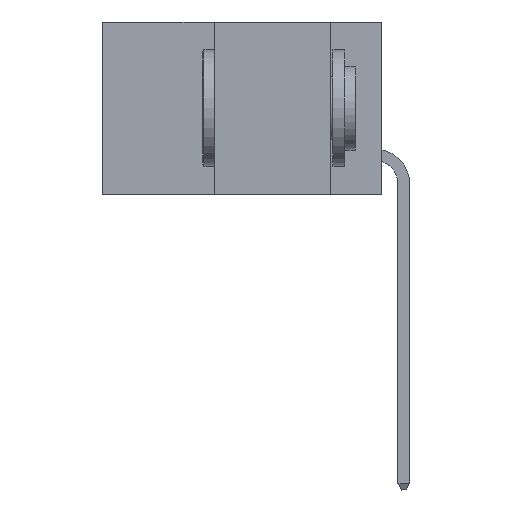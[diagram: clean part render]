
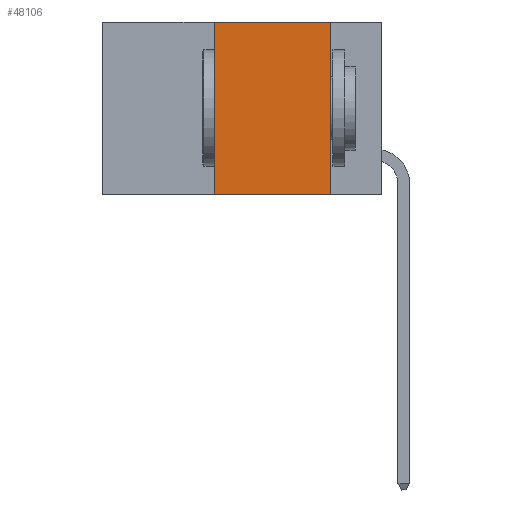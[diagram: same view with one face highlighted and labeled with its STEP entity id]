
A CAD part, left-side view. The second image highlights one B-rep face of the part: STEP entity #48106.
In plain terms, the highlighted planar face has unit normal (-1, 0, 0).
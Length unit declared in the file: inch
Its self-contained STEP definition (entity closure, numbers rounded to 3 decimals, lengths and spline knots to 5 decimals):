
#1676 = AXIS2_PLACEMENT_3D ( 'NONE', #21849, #49066, #6400 ) ;
#2608 = CARTESIAN_POINT ( 'NONE',  ( 0., 0.6, 0. ) ) ;
#2931 = EDGE_CURVE ( 'NONE', #5460, #25511, #46771, .T. ) ;
#4174 = VECTOR ( 'NONE', #49754, 39.37008 ) ;
#5460 = VERTEX_POINT ( 'NONE', #28801 ) ;
#6400 = DIRECTION ( 'NONE',  ( 0., 0., -1. ) ) ;
#6479 = LINE ( 'NONE', #19989, #36795 ) ;
#8018 = VECTOR ( 'NONE', #45074, 39.37008 ) ;
#8444 = EDGE_LOOP ( 'NONE', ( #31469, #32589, #28650, #41458 ) ) ;
#11286 = EDGE_CURVE ( 'NONE', #25511, #27741, #6479, .T. ) ;
#11291 = CARTESIAN_POINT ( 'NONE',  ( 0., 0.36, 0. ) ) ;
#11582 = FACE_OUTER_BOUND ( 'NONE', #8444, .T. ) ;
#19398 = LINE ( 'NONE', #11291, #4174 ) ;
#19742 = EDGE_CURVE ( 'NONE', #22829, #27741, #23782, .T. ) ;
#19989 = CARTESIAN_POINT ( 'NONE',  ( 0., 0.11, 0. ) ) ;
#20583 = CARTESIAN_POINT ( 'NONE',  ( 0., 0.11, 0. ) ) ;
#20802 = DIRECTION ( 'NONE',  ( 0., 0., -1. ) ) ;
#21849 = CARTESIAN_POINT ( 'NONE',  ( 0., 0.6, 0. ) ) ;
#21860 = VECTOR ( 'NONE', #29839, 39.37008 ) ;
#22829 = VERTEX_POINT ( 'NONE', #43567 ) ;
#23782 = LINE ( 'NONE', #48353, #8018 ) ;
#25511 = VERTEX_POINT ( 'NONE', #20583 ) ;
#27741 = VERTEX_POINT ( 'NONE', #35866 ) ;
#28650 = ORIENTED_EDGE ( 'NONE', *, *, #49123, .F. ) ;
#28801 = CARTESIAN_POINT ( 'NONE',  ( 0., 0.36, 0. ) ) ;
#29839 = DIRECTION ( 'NONE',  ( 0., -1., 0. ) ) ;
#31469 = ORIENTED_EDGE ( 'NONE', *, *, #11286, .F. ) ;
#32589 = ORIENTED_EDGE ( 'NONE', *, *, #2931, .F. ) ;
#32850 = PLANE ( 'NONE',  #1676 ) ;
#35866 = CARTESIAN_POINT ( 'NONE',  ( 0., 0.11, -0.37 ) ) ;
#36795 = VECTOR ( 'NONE', #20802, 39.37008 ) ;
#41458 = ORIENTED_EDGE ( 'NONE', *, *, #19742, .T. ) ;
#43567 = CARTESIAN_POINT ( 'NONE',  ( 0., 0.36, -0.37 ) ) ;
#45074 = DIRECTION ( 'NONE',  ( 0., -1., 0. ) ) ;
#46771 = LINE ( 'NONE', #2608, #21860 ) ;
#48106 = ADVANCED_FACE ( 'NONE', ( #11582 ), #32850, .F. ) ;
#48353 = CARTESIAN_POINT ( 'NONE',  ( 0., 0.6, -0.37 ) ) ;
#49066 = DIRECTION ( 'NONE',  ( 1., 0., 0. ) ) ;
#49123 = EDGE_CURVE ( 'NONE', #22829, #5460, #19398, .T. ) ;
#49754 = DIRECTION ( 'NONE',  ( 0., 0., 1. ) ) ;
